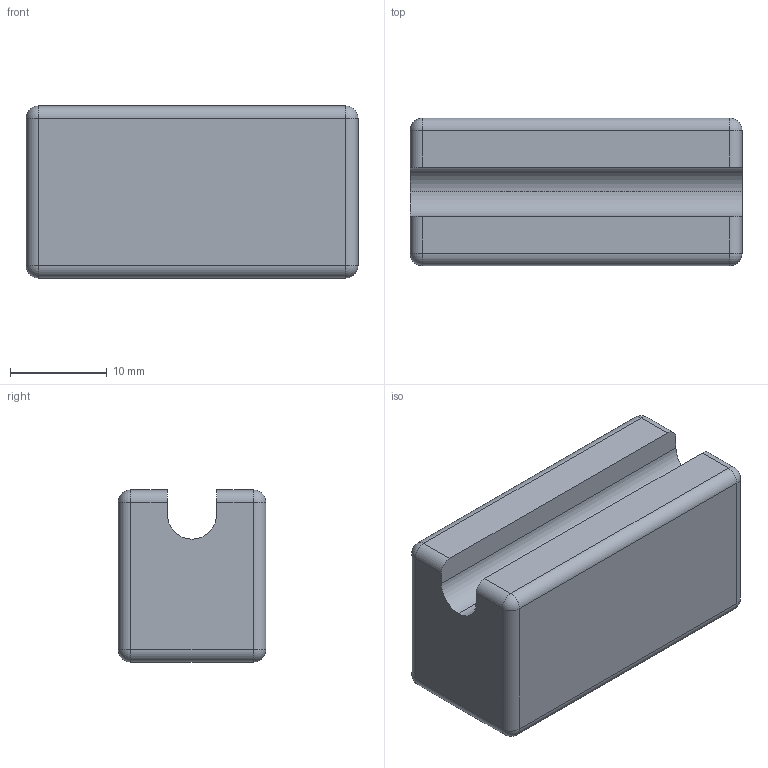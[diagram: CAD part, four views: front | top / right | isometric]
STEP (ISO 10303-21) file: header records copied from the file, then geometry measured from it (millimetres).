
FILE_DESCRIPTION (( 'STEP AP214' ), '1' );
FILE_NAME ('follower.STEP', '2013-11-06T01:48:14', ( '' ), ( '' ), 'SwSTEP 2.0', 'SolidWorks 2013', '' );
FILE_SCHEMA (( 'AUTOMOTIVE_DESIGN' ));
Length unit declared in the file: inch
Products named in the file (1): follower
Bounding box: 34.29 x 15.24 x 17.78 mm (x, y, z)
Volume: 8405.9 mm3; surface area: 2936.2 mm2
Topology: 1 solids, 1 shells, 82 faces, 209 edges, 126 vertices
Faces by surface type: plane 29, bspline 29, cylinder 16, sphere 8
Entity records: 4207 total; most frequent: CARTESIAN_POINT 2415, ORIENTED_EDGE 402, DIRECTION 283, EDGE_CURVE 201, VERTEX_POINT 126, VECTOR 111, LINE 111, EDGE_LOOP 87
